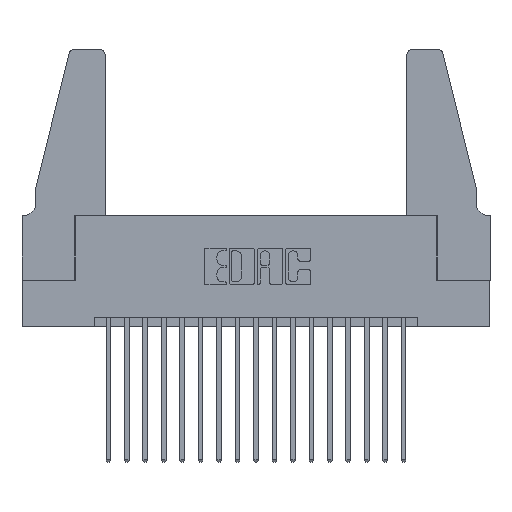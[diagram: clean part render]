
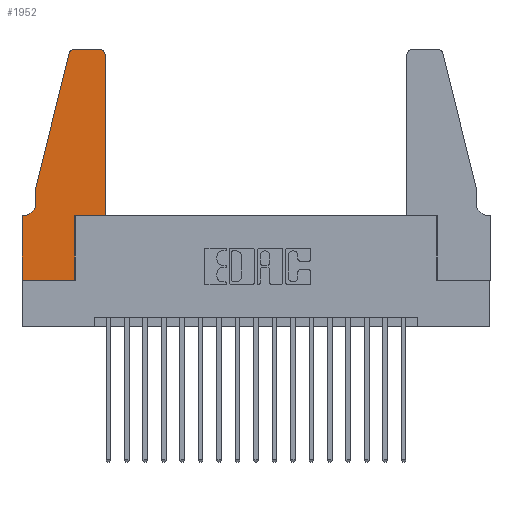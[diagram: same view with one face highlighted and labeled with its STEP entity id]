
A CAD part, top view. The second image highlights one B-rep face of the part: STEP entity #1952.
In plain terms, the highlighted planar face has unit normal (0, 0, 1).
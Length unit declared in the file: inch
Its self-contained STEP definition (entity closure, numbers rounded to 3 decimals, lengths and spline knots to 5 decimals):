
#1 = DIRECTION ( 'NONE',  ( 0., 1., 0. ) ) ;
#29 = VECTOR ( 'NONE', #9315, 39.37008 ) ;
#105 = DIRECTION ( 'NONE',  ( 1., 0., 0. ) ) ;
#154 = CARTESIAN_POINT ( 'NONE',  ( 0.4205, 1.25, 0.37 ) ) ;
#816 = EDGE_CURVE ( 'NONE', #8619, #14746, #1455, .T. ) ;
#893 = LINE ( 'NONE', #5904, #11849 ) ;
#1287 = CARTESIAN_POINT ( 'NONE',  ( 0.2865, 0.35, 0.37 ) ) ;
#1386 = CARTESIAN_POINT ( 'NONE',  ( 0., 0.35, 0.37 ) ) ;
#1455 = LINE ( 'NONE', #11153, #16131 ) ;
#1531 = CARTESIAN_POINT ( 'NONE',  ( 0.4205, 1.22, 0.37 ) ) ;
#1952 = ADVANCED_FACE ( 'NONE', ( #12369 ), #16012, .T. ) ;
#2425 = CARTESIAN_POINT ( 'NONE',  ( 0.4505, 0.35, 0.37 ) ) ;
#2469 = VECTOR ( 'NONE', #5599, 39.37008 ) ;
#2679 = EDGE_CURVE ( 'NONE', #14746, #11855, #11679, .T. ) ;
#2737 = VERTEX_POINT ( 'NONE', #6251 ) ;
#2761 = ORIENTED_EDGE ( 'NONE', *, *, #2679, .T. ) ;
#3030 = DIRECTION ( 'NONE',  ( 1., 0., 0. ) ) ;
#3096 = AXIS2_PLACEMENT_3D ( 'NONE', #1386, #13236, #4380 ) ;
#3252 = LINE ( 'NONE', #8837, #3720 ) ;
#3503 = CARTESIAN_POINT ( 'NONE',  ( 0.4505, 0.35, 0.37 ) ) ;
#3642 = DIRECTION ( 'NONE',  ( 0., -1., 0. ) ) ;
#3720 = VECTOR ( 'NONE', #17409, 39.37008 ) ;
#3764 = CARTESIAN_POINT ( 'NONE',  ( 0.0055, 0.35, 0.37 ) ) ;
#3767 = VECTOR ( 'NONE', #7272, 39.37008 ) ;
#3805 = EDGE_CURVE ( 'NONE', #13204, #2737, #893, .T. ) ;
#4232 = DIRECTION ( 'NONE',  ( 0., 0., -1. ) ) ;
#4380 = DIRECTION ( 'NONE',  ( 1., 0., 0. ) ) ;
#4383 = VERTEX_POINT ( 'NONE', #18635 ) ;
#4415 = EDGE_CURVE ( 'NONE', #4383, #4753, #10694, .T. ) ;
#4753 = VERTEX_POINT ( 'NONE', #3764 ) ;
#4835 = CARTESIAN_POINT ( 'NONE',  ( 0.0755, 0.5, 0.37 ) ) ;
#4967 = CARTESIAN_POINT ( 'NONE',  ( 0.0755, 0.5, 0.37 ) ) ;
#5030 = DIRECTION ( 'NONE',  ( 1., 0., 0. ) ) ;
#5035 = ORIENTED_EDGE ( 'NONE', *, *, #18539, .T. ) ;
#5599 = DIRECTION ( 'NONE',  ( 1., 0., 0. ) ) ;
#5612 = EDGE_CURVE ( 'NONE', #7283, #11751, #6912, .T. ) ;
#5640 = VECTOR ( 'NONE', #5030, 39.37008 ) ;
#5895 = CIRCLE ( 'NONE', #16902, 0.03 ) ;
#5904 = CARTESIAN_POINT ( 'NONE',  ( 0.4505, 0.35, 0.37 ) ) ;
#6107 = ORIENTED_EDGE ( 'NONE', *, *, #15014, .T. ) ;
#6251 = CARTESIAN_POINT ( 'NONE',  ( 0.4505, 1.22, 0.37 ) ) ;
#6650 = ORIENTED_EDGE ( 'NONE', *, *, #5612, .T. ) ;
#6912 = LINE ( 'NONE', #17195, #2469 ) ;
#7001 = LINE ( 'NONE', #4835, #14335 ) ;
#7272 = DIRECTION ( 'NONE',  ( 0., -1., 0. ) ) ;
#7283 = VERTEX_POINT ( 'NONE', #8025 ) ;
#7502 = LINE ( 'NONE', #16443, #29 ) ;
#7778 = EDGE_LOOP ( 'NONE', ( #10376, #2761, #6107, #17091, #9407, #5035, #14257, #6650, #18470, #9581, #13962, #15763 ) ) ;
#7962 = DIRECTION ( 'NONE',  ( -1., 0., 0. ) ) ;
#8025 = CARTESIAN_POINT ( 'NONE',  ( 0., 0., 0.37 ) ) ;
#8101 = EDGE_CURVE ( 'NONE', #10459, #13204, #13475, .T. ) ;
#8243 = LINE ( 'NONE', #17373, #3767 ) ;
#8619 = VERTEX_POINT ( 'NONE', #154 ) ;
#8655 = AXIS2_PLACEMENT_3D ( 'NONE', #17648, #9080, #105 ) ;
#8837 = CARTESIAN_POINT ( 'NONE',  ( 0.2865, 0.35, 0.37 ) ) ;
#9080 = DIRECTION ( 'NONE',  ( 0., 0., 1. ) ) ;
#9315 = DIRECTION ( 'NONE',  ( -1., 0., 0. ) ) ;
#9407 = ORIENTED_EDGE ( 'NONE', *, *, #4415, .T. ) ;
#9581 = ORIENTED_EDGE ( 'NONE', *, *, #8101, .T. ) ;
#10376 = ORIENTED_EDGE ( 'NONE', *, *, #816, .T. ) ;
#10459 = VERTEX_POINT ( 'NONE', #1287 ) ;
#10694 = CIRCLE ( 'NONE', #12708, 0.07 ) ;
#11153 = CARTESIAN_POINT ( 'NONE',  ( 0.2605, 1.25, 0.37 ) ) ;
#11243 = EDGE_CURVE ( 'NONE', #17608, #7283, #11806, .T. ) ;
#11363 = CARTESIAN_POINT ( 'NONE',  ( 0., 0.35, 0.37 ) ) ;
#11679 = CIRCLE ( 'NONE', #8655, 0.03 ) ;
#11751 = VERTEX_POINT ( 'NONE', #12266 ) ;
#11806 = LINE ( 'NONE', #12533, #15132 ) ;
#11849 = VECTOR ( 'NONE', #1, 39.37008 ) ;
#11855 = VERTEX_POINT ( 'NONE', #13901 ) ;
#11948 = DIRECTION ( 'NONE',  ( 0., 0., 1. ) ) ;
#12266 = CARTESIAN_POINT ( 'NONE',  ( 0.2865, 0., 0.37 ) ) ;
#12369 = FACE_OUTER_BOUND ( 'NONE', #7778, .T. ) ;
#12533 = CARTESIAN_POINT ( 'NONE',  ( 0., 0., 0.37 ) ) ;
#12708 = AXIS2_PLACEMENT_3D ( 'NONE', #13107, #4232, #14522 ) ;
#13107 = CARTESIAN_POINT ( 'NONE',  ( 0.0055, 0.42, 0.37 ) ) ;
#13204 = VERTEX_POINT ( 'NONE', #2425 ) ;
#13236 = DIRECTION ( 'NONE',  ( 0., 0., 1. ) ) ;
#13475 = LINE ( 'NONE', #3503, #5640 ) ;
#13901 = CARTESIAN_POINT ( 'NONE',  ( 0.25487, 1.22718, 0.37 ) ) ;
#13962 = ORIENTED_EDGE ( 'NONE', *, *, #3805, .T. ) ;
#14257 = ORIENTED_EDGE ( 'NONE', *, *, #11243, .T. ) ;
#14335 = VECTOR ( 'NONE', #17911, 39.37008 ) ;
#14522 = DIRECTION ( 'NONE',  ( -1., 0., 0. ) ) ;
#14746 = VERTEX_POINT ( 'NONE', #17288 ) ;
#14799 = EDGE_CURVE ( 'NONE', #11751, #10459, #3252, .T. ) ;
#15014 = EDGE_CURVE ( 'NONE', #11855, #17515, #7001, .T. ) ;
#15132 = VECTOR ( 'NONE', #3642, 39.37008 ) ;
#15763 = ORIENTED_EDGE ( 'NONE', *, *, #18401, .T. ) ;
#16012 = PLANE ( 'NONE',  #3096 ) ;
#16131 = VECTOR ( 'NONE', #7962, 39.37008 ) ;
#16443 = CARTESIAN_POINT ( 'NONE',  ( 0.0755, 0.35, 0.37 ) ) ;
#16902 = AXIS2_PLACEMENT_3D ( 'NONE', #1531, #11948, #3030 ) ;
#17091 = ORIENTED_EDGE ( 'NONE', *, *, #18321, .T. ) ;
#17195 = CARTESIAN_POINT ( 'NONE',  ( 0., 0., 0.37 ) ) ;
#17288 = CARTESIAN_POINT ( 'NONE',  ( 0.284, 1.25, 0.37 ) ) ;
#17373 = CARTESIAN_POINT ( 'NONE',  ( 0.0755, 0.5, 0.37 ) ) ;
#17409 = DIRECTION ( 'NONE',  ( 0., 1., 0. ) ) ;
#17515 = VERTEX_POINT ( 'NONE', #4967 ) ;
#17608 = VERTEX_POINT ( 'NONE', #11363 ) ;
#17648 = CARTESIAN_POINT ( 'NONE',  ( 0.284, 1.22, 0.37 ) ) ;
#17911 = DIRECTION ( 'NONE',  ( -0.239, -0.971, 0. ) ) ;
#18321 = EDGE_CURVE ( 'NONE', #17515, #4383, #8243, .T. ) ;
#18401 = EDGE_CURVE ( 'NONE', #2737, #8619, #5895, .T. ) ;
#18470 = ORIENTED_EDGE ( 'NONE', *, *, #14799, .T. ) ;
#18539 = EDGE_CURVE ( 'NONE', #4753, #17608, #7502, .T. ) ;
#18635 = CARTESIAN_POINT ( 'NONE',  ( 0.0755, 0.42, 0.37 ) ) ;
